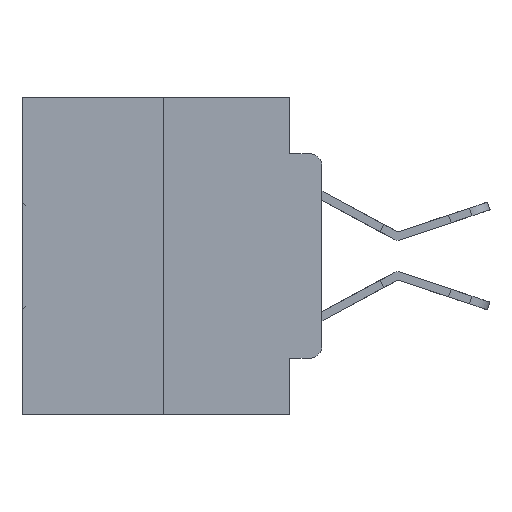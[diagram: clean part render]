
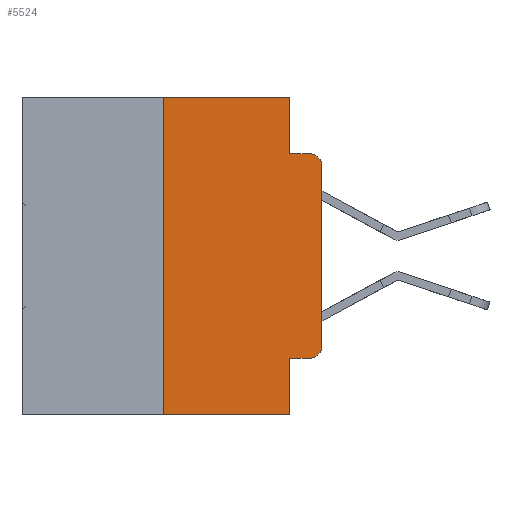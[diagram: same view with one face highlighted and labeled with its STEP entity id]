
A CAD part, left-side view. The second image highlights one B-rep face of the part: STEP entity #5524.
In plain terms, the highlighted planar face has unit normal (-1, 0, 0).
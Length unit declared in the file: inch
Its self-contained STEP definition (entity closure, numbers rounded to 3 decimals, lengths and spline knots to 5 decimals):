
#192 = PLANE ( 'NONE',  #7971 ) ;
#1009 = CARTESIAN_POINT ( 'NONE',  ( 0., 0.473, 0. ) ) ;
#1017 = EDGE_CURVE ( 'NONE', #29991, #8128, #27794, .T. ) ;
#4043 = LINE ( 'NONE', #19595, #17212 ) ;
#4284 = EDGE_CURVE ( 'NONE', #16117, #16967, #18520, .T. ) ;
#4932 = EDGE_CURVE ( 'NONE', #11770, #16967, #4043, .T. ) ;
#5524 = ADVANCED_FACE ( 'NONE', ( #26287 ), #192, .F. ) ;
#5657 = EDGE_CURVE ( 'NONE', #32956, #7747, #15108, .T. ) ;
#5963 = DIRECTION ( 'NONE',  ( -1., 0., 0. ) ) ;
#5998 = LINE ( 'NONE', #9072, #33240 ) ;
#6388 = DIRECTION ( 'NONE',  ( 0., 0., 1. ) ) ;
#7067 = VECTOR ( 'NONE', #20308, 39.37008 ) ;
#7144 = CARTESIAN_POINT ( 'NONE',  ( 0., 0., -0.1085 ) ) ;
#7426 = VERTEX_POINT ( 'NONE', #21557 ) ;
#7747 = VERTEX_POINT ( 'NONE', #33402 ) ;
#7971 = AXIS2_PLACEMENT_3D ( 'NONE', #23886, #8050, #26535 ) ;
#8050 = DIRECTION ( 'NONE',  ( 1., 0., 0. ) ) ;
#8128 = VERTEX_POINT ( 'NONE', #27513 ) ;
#8544 = DIRECTION ( 'NONE',  ( 0., -1., 0. ) ) ;
#8894 = DIRECTION ( 'NONE',  ( 0., -1., 0. ) ) ;
#9041 = ORIENTED_EDGE ( 'NONE', *, *, #18000, .T. ) ;
#9042 = CARTESIAN_POINT ( 'NONE',  ( 0., 0., 0. ) ) ;
#9065 = CARTESIAN_POINT ( 'NONE',  ( 0., 0.051, -0.4115 ) ) ;
#9072 = CARTESIAN_POINT ( 'NONE',  ( 0., 0.25, 0. ) ) ;
#9347 = EDGE_CURVE ( 'NONE', #29563, #17269, #12977, .T. ) ;
#10055 = CARTESIAN_POINT ( 'NONE',  ( 0., 0.25, -0.5 ) ) ;
#10447 = ORIENTED_EDGE ( 'NONE', *, *, #1017, .F. ) ;
#10659 = VECTOR ( 'NONE', #8544, 39.37008 ) ;
#10687 = ORIENTED_EDGE ( 'NONE', *, *, #23857, .F. ) ;
#11184 = CARTESIAN_POINT ( 'NONE',  ( 0., 0.473, -0.5 ) ) ;
#11363 = CARTESIAN_POINT ( 'NONE',  ( 0., 0.02, -0.1085 ) ) ;
#11770 = VERTEX_POINT ( 'NONE', #9065 ) ;
#12430 = VECTOR ( 'NONE', #8894, 39.37008 ) ;
#12667 = VECTOR ( 'NONE', #6388, 39.37008 ) ;
#12977 = CIRCLE ( 'NONE', #24887, 0.02 ) ;
#13498 = DIRECTION ( 'NONE',  ( 0., -1., 0. ) ) ;
#13846 = CARTESIAN_POINT ( 'NONE',  ( 0., 0.02, -0.4115 ) ) ;
#13944 = ORIENTED_EDGE ( 'NONE', *, *, #9347, .T. ) ;
#14009 = DIRECTION ( 'NONE',  ( 0., 0., -1. ) ) ;
#14231 = ORIENTED_EDGE ( 'NONE', *, *, #4932, .F. ) ;
#15062 = AXIS2_PLACEMENT_3D ( 'NONE', #21788, #5963, #24444 ) ;
#15108 = CIRCLE ( 'NONE', #15062, 0.02 ) ;
#16117 = VERTEX_POINT ( 'NONE', #10055 ) ;
#16271 = VECTOR ( 'NONE', #13498, 39.37008 ) ;
#16967 = VERTEX_POINT ( 'NONE', #29153 ) ;
#17212 = VECTOR ( 'NONE', #22280, 39.37008 ) ;
#17269 = VERTEX_POINT ( 'NONE', #27863 ) ;
#18000 = EDGE_CURVE ( 'NONE', #11770, #32956, #26478, .T. ) ;
#18439 = DIRECTION ( 'NONE',  ( 0., 0., -1. ) ) ;
#18520 = LINE ( 'NONE', #11184, #10659 ) ;
#19360 = ORIENTED_EDGE ( 'NONE', *, *, #19652, .F. ) ;
#19468 = LINE ( 'NONE', #1009, #12430 ) ;
#19595 = CARTESIAN_POINT ( 'NONE',  ( 0., 0.051, 0. ) ) ;
#19652 = EDGE_CURVE ( 'NONE', #7426, #29991, #19468, .T. ) ;
#20308 = DIRECTION ( 'NONE',  ( 0., -1., 0. ) ) ;
#20755 = VECTOR ( 'NONE', #18439, 39.37008 ) ;
#20797 = ORIENTED_EDGE ( 'NONE', *, *, #30540, .T. ) ;
#21557 = CARTESIAN_POINT ( 'NONE',  ( 0., 0.25, 0. ) ) ;
#21788 = CARTESIAN_POINT ( 'NONE',  ( 0., 0.02, -0.3915 ) ) ;
#22280 = DIRECTION ( 'NONE',  ( 0., 0., -1. ) ) ;
#23857 = EDGE_CURVE ( 'NONE', #16117, #7426, #5998, .T. ) ;
#23886 = CARTESIAN_POINT ( 'NONE',  ( 0., 0.473, 0. ) ) ;
#24444 = DIRECTION ( 'NONE',  ( 0., 0., -1. ) ) ;
#24887 = AXIS2_PLACEMENT_3D ( 'NONE', #11363, #29846, #14009 ) ;
#25690 = EDGE_CURVE ( 'NONE', #8128, #17269, #31155, .T. ) ;
#26287 = FACE_OUTER_BOUND ( 'NONE', #32265, .T. ) ;
#26478 = LINE ( 'NONE', #33423, #7067 ) ;
#26535 = DIRECTION ( 'NONE',  ( 0., 0., -1. ) ) ;
#26737 = LINE ( 'NONE', #9042, #12667 ) ;
#27513 = CARTESIAN_POINT ( 'NONE',  ( 0., 0.051, -0.0885 ) ) ;
#27794 = LINE ( 'NONE', #32311, #20755 ) ;
#27863 = CARTESIAN_POINT ( 'NONE',  ( 0., 0.02, -0.0885 ) ) ;
#29153 = CARTESIAN_POINT ( 'NONE',  ( 0., 0.051, -0.5 ) ) ;
#29563 = VERTEX_POINT ( 'NONE', #7144 ) ;
#29846 = DIRECTION ( 'NONE',  ( -1., 0., 0. ) ) ;
#29991 = VERTEX_POINT ( 'NONE', #30547 ) ;
#30316 = DIRECTION ( 'NONE',  ( 0., 0., 1. ) ) ;
#30501 = ORIENTED_EDGE ( 'NONE', *, *, #5657, .T. ) ;
#30540 = EDGE_CURVE ( 'NONE', #7747, #29563, #26737, .T. ) ;
#30547 = CARTESIAN_POINT ( 'NONE',  ( 0., 0.051, 0. ) ) ;
#31155 = LINE ( 'NONE', #31972, #16271 ) ;
#31319 = ORIENTED_EDGE ( 'NONE', *, *, #4284, .T. ) ;
#31972 = CARTESIAN_POINT ( 'NONE',  ( 0., 0.051, -0.0885 ) ) ;
#32265 = EDGE_LOOP ( 'NONE', ( #20797, #13944, #33734, #10447, #19360, #10687, #31319, #14231, #9041, #30501 ) ) ;
#32311 = CARTESIAN_POINT ( 'NONE',  ( 0., 0.051, 0. ) ) ;
#32956 = VERTEX_POINT ( 'NONE', #13846 ) ;
#33240 = VECTOR ( 'NONE', #30316, 39.37008 ) ;
#33402 = CARTESIAN_POINT ( 'NONE',  ( 0., 0., -0.3915 ) ) ;
#33423 = CARTESIAN_POINT ( 'NONE',  ( 0., 0.051, -0.4115 ) ) ;
#33734 = ORIENTED_EDGE ( 'NONE', *, *, #25690, .F. ) ;
